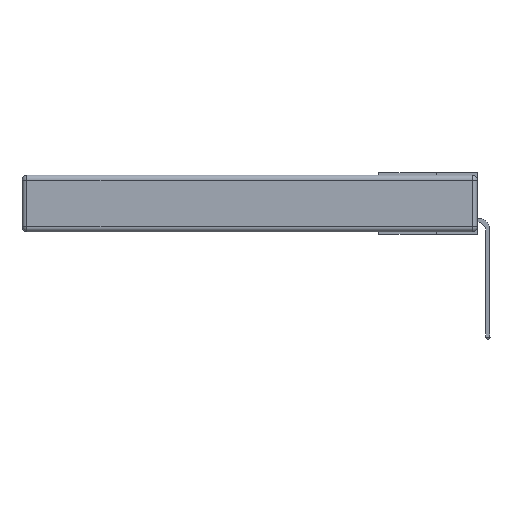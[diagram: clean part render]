
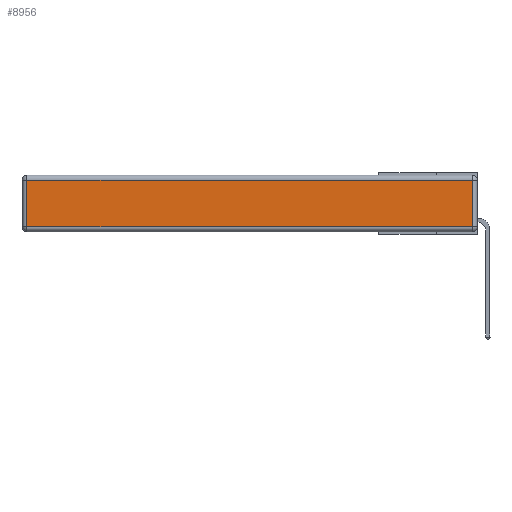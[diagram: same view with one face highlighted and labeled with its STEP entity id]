
A CAD part, left-side view. The second image highlights one B-rep face of the part: STEP entity #8956.
In plain terms, the highlighted planar face has unit normal (-1, 0, 0).
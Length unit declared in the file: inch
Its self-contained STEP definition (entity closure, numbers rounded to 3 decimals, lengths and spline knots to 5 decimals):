
#504 = DIRECTION ( 'NONE',  ( 0., 1., 0. ) ) ;
#598 = DIRECTION ( 'NONE',  ( 0., 0., -1. ) ) ;
#716 = EDGE_CURVE ( 'NONE', #2002, #2476, #2100, .T. ) ;
#839 = EDGE_LOOP ( 'NONE', ( #7351, #4701, #1916, #5825 ) ) ;
#993 = AXIS2_PLACEMENT_3D ( 'NONE', #3537, #5114, #3107 ) ;
#1289 = CARTESIAN_POINT ( 'NONE',  ( 0., 2.72, -0.343 ) ) ;
#1344 = VECTOR ( 'NONE', #5040, 39.37008 ) ;
#1916 = ORIENTED_EDGE ( 'NONE', *, *, #8180, .T. ) ;
#2002 = VERTEX_POINT ( 'NONE', #10439 ) ;
#2062 = CARTESIAN_POINT ( 'NONE',  ( 0., 0.03, -0.03 ) ) ;
#2100 = LINE ( 'NONE', #12086, #4974 ) ;
#2399 = LINE ( 'NONE', #10034, #1344 ) ;
#2476 = VERTEX_POINT ( 'NONE', #5872 ) ;
#2527 = PLANE ( 'NONE',  #993 ) ;
#3107 = DIRECTION ( 'NONE',  ( 0., 0., 1. ) ) ;
#3148 = VERTEX_POINT ( 'NONE', #2062 ) ;
#3537 = CARTESIAN_POINT ( 'NONE',  ( 0., 0., -0.343 ) ) ;
#3833 = VERTEX_POINT ( 'NONE', #8816 ) ;
#4668 = EDGE_CURVE ( 'NONE', #3833, #2002, #11084, .T. ) ;
#4701 = ORIENTED_EDGE ( 'NONE', *, *, #11609, .T. ) ;
#4974 = VECTOR ( 'NONE', #10095, 39.37008 ) ;
#5040 = DIRECTION ( 'NONE',  ( 0., 0., 1. ) ) ;
#5114 = DIRECTION ( 'NONE',  ( -1., 0., 0. ) ) ;
#5206 = FACE_OUTER_BOUND ( 'NONE', #839, .T. ) ;
#5825 = ORIENTED_EDGE ( 'NONE', *, *, #4668, .T. ) ;
#5872 = CARTESIAN_POINT ( 'NONE',  ( 0., 0.03, -0.313 ) ) ;
#7123 = VECTOR ( 'NONE', #598, 39.37008 ) ;
#7351 = ORIENTED_EDGE ( 'NONE', *, *, #716, .T. ) ;
#8180 = EDGE_CURVE ( 'NONE', #3148, #3833, #12380, .T. ) ;
#8375 = CARTESIAN_POINT ( 'NONE',  ( 0., 2.75, -0.03 ) ) ;
#8816 = CARTESIAN_POINT ( 'NONE',  ( 0., 2.72, -0.03 ) ) ;
#8956 = ADVANCED_FACE ( 'NONE', ( #5206 ), #2527, .T. ) ;
#10034 = CARTESIAN_POINT ( 'NONE',  ( 0., 0.03, -0.343 ) ) ;
#10095 = DIRECTION ( 'NONE',  ( 0., -1., 0. ) ) ;
#10439 = CARTESIAN_POINT ( 'NONE',  ( 0., 2.72, -0.313 ) ) ;
#11084 = LINE ( 'NONE', #1289, #7123 ) ;
#11609 = EDGE_CURVE ( 'NONE', #2476, #3148, #2399, .T. ) ;
#12086 = CARTESIAN_POINT ( 'NONE',  ( 0., 0., -0.313 ) ) ;
#12380 = LINE ( 'NONE', #8375, #12525 ) ;
#12525 = VECTOR ( 'NONE', #504, 39.37008 ) ;
